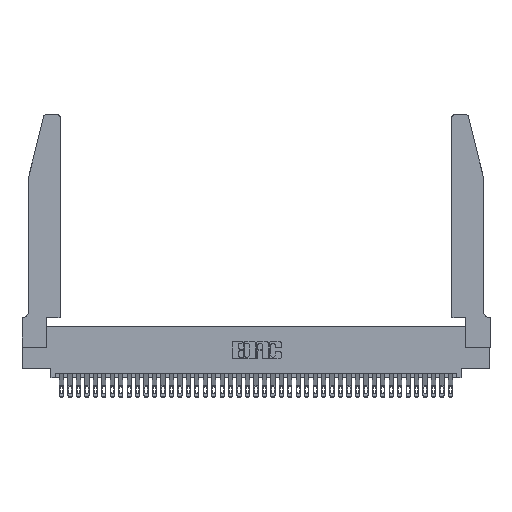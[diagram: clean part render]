
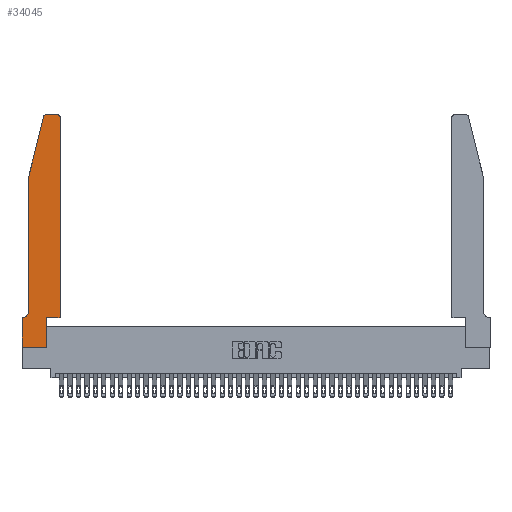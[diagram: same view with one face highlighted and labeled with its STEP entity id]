
A CAD part, top view. The second image highlights one B-rep face of the part: STEP entity #34045.
In plain terms, the highlighted planar face has unit normal (0, 0, 1).
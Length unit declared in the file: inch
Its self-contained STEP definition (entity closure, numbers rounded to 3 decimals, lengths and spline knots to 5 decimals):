
#646 = LINE ( 'NONE', #34848, #40199 ) ;
#1281 = ORIENTED_EDGE ( 'NONE', *, *, #31990, .T. ) ;
#1554 = CARTESIAN_POINT ( 'NONE',  ( 0.0755, 0.35, 0.37 ) ) ;
#1621 = DIRECTION ( 'NONE',  ( 0., 0., 1. ) ) ;
#1818 = DIRECTION ( 'NONE',  ( 0., 1., 0. ) ) ;
#2331 = CARTESIAN_POINT ( 'NONE',  ( 0.4505, 2.72, 0.37 ) ) ;
#2929 = VERTEX_POINT ( 'NONE', #15228 ) ;
#4337 = LINE ( 'NONE', #19054, #37387 ) ;
#4785 = DIRECTION ( 'NONE',  ( -1., 0., 0. ) ) ;
#6000 = LINE ( 'NONE', #16562, #38013 ) ;
#6266 = EDGE_CURVE ( 'NONE', #13959, #32758, #10439, .T. ) ;
#6300 = DIRECTION ( 'NONE',  ( 0., 0., 1. ) ) ;
#6326 = DIRECTION ( 'NONE',  ( 0., 1., 0. ) ) ;
#8502 = CARTESIAN_POINT ( 'NONE',  ( 0.284, 2.72, 0.37 ) ) ;
#8704 = EDGE_CURVE ( 'NONE', #21957, #13959, #26294, .T. ) ;
#8977 = VERTEX_POINT ( 'NONE', #28018 ) ;
#8984 = AXIS2_PLACEMENT_3D ( 'NONE', #17199, #39568, #20434 ) ;
#9382 = VECTOR ( 'NONE', #17428, 39.37008 ) ;
#9717 = VERTEX_POINT ( 'NONE', #38813 ) ;
#10439 = LINE ( 'NONE', #17755, #35983 ) ;
#11346 = ORIENTED_EDGE ( 'NONE', *, *, #18207, .T. ) ;
#11476 = ORIENTED_EDGE ( 'NONE', *, *, #24679, .T. ) ;
#11582 = EDGE_LOOP ( 'NONE', ( #13504, #33079, #17892, #11346, #39369, #11476, #12337, #20391, #25354, #1281, #13481, #40098 ) ) ;
#11677 = DIRECTION ( 'NONE',  ( 1., 0., 0. ) ) ;
#12337 = ORIENTED_EDGE ( 'NONE', *, *, #15144, .T. ) ;
#13004 = CIRCLE ( 'NONE', #23124, 0.03 ) ;
#13481 = ORIENTED_EDGE ( 'NONE', *, *, #38609, .T. ) ;
#13504 = ORIENTED_EDGE ( 'NONE', *, *, #6266, .T. ) ;
#13581 = CARTESIAN_POINT ( 'NONE',  ( 0.4505, 0.35, 0.37 ) ) ;
#13881 = VERTEX_POINT ( 'NONE', #23265 ) ;
#13959 = VERTEX_POINT ( 'NONE', #33012 ) ;
#14206 = CARTESIAN_POINT ( 'NONE',  ( 0., 0., 0.37 ) ) ;
#14679 = FACE_OUTER_BOUND ( 'NONE', #11582, .T. ) ;
#15144 = EDGE_CURVE ( 'NONE', #40125, #22470, #6000, .T. ) ;
#15228 = CARTESIAN_POINT ( 'NONE',  ( 0.4505, 0.35, 0.37 ) ) ;
#16364 = VECTOR ( 'NONE', #32748, 39.37008 ) ;
#16455 = VECTOR ( 'NONE', #33585, 39.37008 ) ;
#16562 = CARTESIAN_POINT ( 'NONE',  ( 0., 0., 0.37 ) ) ;
#16615 = EDGE_CURVE ( 'NONE', #22470, #28395, #34903, .T. ) ;
#16872 = VECTOR ( 'NONE', #1818, 39.37008 ) ;
#17199 = CARTESIAN_POINT ( 'NONE',  ( 0.0055, 0.42, 0.37 ) ) ;
#17364 = LINE ( 'NONE', #13581, #16364 ) ;
#17424 = AXIS2_PLACEMENT_3D ( 'NONE', #25484, #6300, #28693 ) ;
#17428 = DIRECTION ( 'NONE',  ( 1., 0., 0. ) ) ;
#17632 = LINE ( 'NONE', #1554, #25163 ) ;
#17755 = CARTESIAN_POINT ( 'NONE',  ( 0.2605, 2.75, 0.37 ) ) ;
#17885 = LINE ( 'NONE', #33704, #16872 ) ;
#17892 = ORIENTED_EDGE ( 'NONE', *, *, #34024, .T. ) ;
#18207 = EDGE_CURVE ( 'NONE', #41377, #8977, #35486, .T. ) ;
#18699 = AXIS2_PLACEMENT_3D ( 'NONE', #20808, #1621, #24049 ) ;
#18844 = CIRCLE ( 'NONE', #8984, 0.07 ) ;
#19054 = CARTESIAN_POINT ( 'NONE',  ( 0.2865, 0.35, 0.37 ) ) ;
#19421 = CARTESIAN_POINT ( 'NONE',  ( 0.284, 2.75, 0.37 ) ) ;
#20391 = ORIENTED_EDGE ( 'NONE', *, *, #16615, .T. ) ;
#20434 = DIRECTION ( 'NONE',  ( -1., 0., 0. ) ) ;
#20808 = CARTESIAN_POINT ( 'NONE',  ( 0.4205, 2.72, 0.37 ) ) ;
#21957 = VERTEX_POINT ( 'NONE', #2331 ) ;
#22470 = VERTEX_POINT ( 'NONE', #27087 ) ;
#23013 = DIRECTION ( 'NONE',  ( 0., -1., 0. ) ) ;
#23124 = AXIS2_PLACEMENT_3D ( 'NONE', #8502, #30854, #11677 ) ;
#23265 = CARTESIAN_POINT ( 'NONE',  ( 0.0055, 0.35, 0.37 ) ) ;
#23981 = CARTESIAN_POINT ( 'NONE',  ( 0.0755, 2., 0.37 ) ) ;
#24049 = DIRECTION ( 'NONE',  ( 1., 0., 0. ) ) ;
#24679 = EDGE_CURVE ( 'NONE', #13881, #40125, #17632, .T. ) ;
#25163 = VECTOR ( 'NONE', #4785, 39.37008 ) ;
#25354 = ORIENTED_EDGE ( 'NONE', *, *, #27889, .T. ) ;
#25484 = CARTESIAN_POINT ( 'NONE',  ( 0., 0.35, 0.37 ) ) ;
#25921 = CARTESIAN_POINT ( 'NONE',  ( 0., 0.35, 0.37 ) ) ;
#25952 = EDGE_CURVE ( 'NONE', #32758, #35089, #13004, .T. ) ;
#26294 = CIRCLE ( 'NONE', #18699, 0.03 ) ;
#27087 = CARTESIAN_POINT ( 'NONE',  ( 0., 0., 0.37 ) ) ;
#27451 = DIRECTION ( 'NONE',  ( -1., 0., 0. ) ) ;
#27512 = CARTESIAN_POINT ( 'NONE',  ( 0.25487, 2.72718, 0.37 ) ) ;
#27889 = EDGE_CURVE ( 'NONE', #28395, #9717, #4337, .T. ) ;
#28018 = CARTESIAN_POINT ( 'NONE',  ( 0.0755, 0.42, 0.37 ) ) ;
#28176 = EDGE_CURVE ( 'NONE', #8977, #13881, #18844, .T. ) ;
#28395 = VERTEX_POINT ( 'NONE', #30910 ) ;
#28693 = DIRECTION ( 'NONE',  ( 1., 0., 0. ) ) ;
#30854 = DIRECTION ( 'NONE',  ( 0., 0., 1. ) ) ;
#30910 = CARTESIAN_POINT ( 'NONE',  ( 0.2865, 0., 0.37 ) ) ;
#31759 = DIRECTION ( 'NONE',  ( -0.239, -0.971, 0. ) ) ;
#31990 = EDGE_CURVE ( 'NONE', #9717, #2929, #17364, .T. ) ;
#32748 = DIRECTION ( 'NONE',  ( 1., 0., 0. ) ) ;
#32758 = VERTEX_POINT ( 'NONE', #19421 ) ;
#33012 = CARTESIAN_POINT ( 'NONE',  ( 0.4205, 2.75, 0.37 ) ) ;
#33079 = ORIENTED_EDGE ( 'NONE', *, *, #25952, .T. ) ;
#33585 = DIRECTION ( 'NONE',  ( 0., -1., 0. ) ) ;
#33704 = CARTESIAN_POINT ( 'NONE',  ( 0.4505, 0.35, 0.37 ) ) ;
#34024 = EDGE_CURVE ( 'NONE', #35089, #41377, #646, .T. ) ;
#34045 = ADVANCED_FACE ( 'NONE', ( #14679 ), #41390, .T. ) ;
#34848 = CARTESIAN_POINT ( 'NONE',  ( 0.0755, 2., 0.37 ) ) ;
#34903 = LINE ( 'NONE', #14206, #9382 ) ;
#35089 = VERTEX_POINT ( 'NONE', #27512 ) ;
#35486 = LINE ( 'NONE', #23981, #16455 ) ;
#35983 = VECTOR ( 'NONE', #27451, 39.37008 ) ;
#37387 = VECTOR ( 'NONE', #6326, 39.37008 ) ;
#38013 = VECTOR ( 'NONE', #23013, 39.37008 ) ;
#38609 = EDGE_CURVE ( 'NONE', #2929, #21957, #17885, .T. ) ;
#38813 = CARTESIAN_POINT ( 'NONE',  ( 0.2865, 0.35, 0.37 ) ) ;
#39369 = ORIENTED_EDGE ( 'NONE', *, *, #28176, .T. ) ;
#39568 = DIRECTION ( 'NONE',  ( 0., 0., -1. ) ) ;
#40098 = ORIENTED_EDGE ( 'NONE', *, *, #8704, .T. ) ;
#40125 = VERTEX_POINT ( 'NONE', #25921 ) ;
#40199 = VECTOR ( 'NONE', #31759, 39.37008 ) ;
#40920 = CARTESIAN_POINT ( 'NONE',  ( 0.0755, 2., 0.37 ) ) ;
#41377 = VERTEX_POINT ( 'NONE', #40920 ) ;
#41390 = PLANE ( 'NONE',  #17424 ) ;
